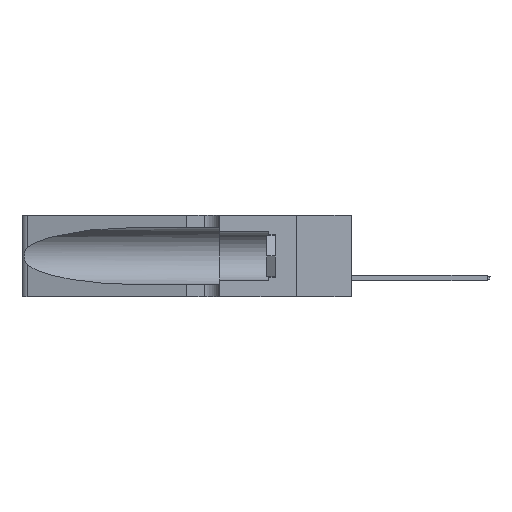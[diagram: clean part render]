
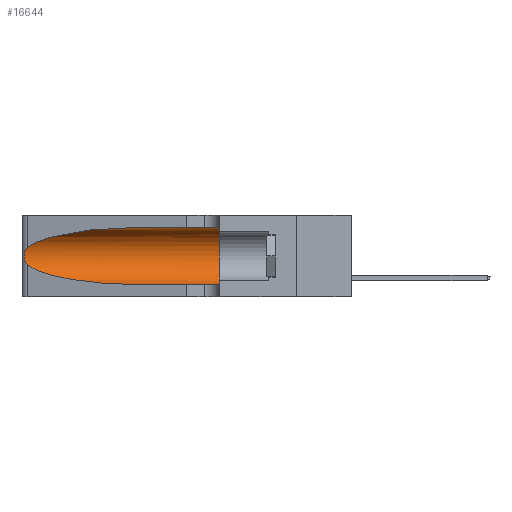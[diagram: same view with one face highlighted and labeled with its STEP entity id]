
A CAD part, left-side view. The second image highlights one B-rep face of the part: STEP entity #16644.
In plain terms, the highlighted cylindrical face has radius 3.308 mm (diameter 6.617 mm), a partial arc.
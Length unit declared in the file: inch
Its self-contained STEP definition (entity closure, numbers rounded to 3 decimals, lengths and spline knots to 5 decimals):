
#372 = CARTESIAN_POINT ( 'NONE',  ( 0.26075, 1.23896, 0.19203 ) ) ;
#516 = CARTESIAN_POINT ( 'NONE',  ( 0.25639, 1.23186, 0.15144 ) ) ;
#840 = ORIENTED_EDGE ( 'NONE', *, *, #10818, .T. ) ;
#975 =( BOUNDED_CURVE ( )  B_SPLINE_CURVE ( 3, ( #2878, #42233, #29083, #22232 ),
 .UNSPECIFIED., .F., .T. ) 
 B_SPLINE_CURVE_WITH_KNOTS ( ( 4, 4 ),
 ( 1.5708, 2.84003 ),
 .UNSPECIFIED. ) 
 CURVE ( )  GEOMETRIC_REPRESENTATION_ITEM ( )  RATIONAL_B_SPLINE_CURVE ( ( 1., 0.87, 0.87, 1. ) ) 
 REPRESENTATION_ITEM ( '' )  );
#1677 = ORIENTED_EDGE ( 'NONE', *, *, #20433, .F. ) ;
#1687 = VERTEX_POINT ( 'NONE', #42105 ) ;
#1975 = EDGE_CURVE ( 'NONE', #4894, #34701, #31952, .T. ) ;
#2878 = CARTESIAN_POINT ( 'NONE',  ( 0.1305, 0.72297, 0.31525 ) ) ;
#3048 = LINE ( 'NONE', #25439, #32761 ) ;
#3253 = CYLINDRICAL_SURFACE ( 'NONE', #29663, 0.13025 ) ;
#4140 = B_SPLINE_CURVE_WITH_KNOTS ( 'NONE', 3,
 ( #6742, #32610, #23046, #16781, #13042, #39171, #372, #6432, #39470, #6877, #10153, #516, #13479, #16913 ),
 .UNSPECIFIED., .F., .F.,
 ( 4, 2, 2, 2, 2, 2, 4 ),
 ( 0., 0.00027, 0.00053, 0.00107, 0.0016, 0.00187, 0.00214 ),
 .UNSPECIFIED. ) ;
#4601 = CARTESIAN_POINT ( 'NONE',  ( 0.25487, 1.22718, 0.14631 ) ) ;
#4681 = CIRCLE ( 'NONE', #40272, 0.13025 ) ;
#4894 = VERTEX_POINT ( 'NONE', #21392 ) ;
#6432 = CARTESIAN_POINT ( 'NONE',  ( 0.26075, 1.23896, 0.178 ) ) ;
#6742 = CARTESIAN_POINT ( 'NONE',  ( 0.25487, 1.22718, 0.22369 ) ) ;
#6877 = CARTESIAN_POINT ( 'NONE',  ( 0.25856, 1.23593, 0.16098 ) ) ;
#10153 = CARTESIAN_POINT ( 'NONE',  ( 0.25789, 1.23486, 0.15765 ) ) ;
#10818 = EDGE_CURVE ( 'NONE', #14510, #4894, #4140, .T. ) ;
#10840 = ORIENTED_EDGE ( 'NONE', *, *, #11871, .T. ) ;
#10971 = CARTESIAN_POINT ( 'NONE',  ( 0.1305, 1.61858, 0.05475 ) ) ;
#11411 = CARTESIAN_POINT ( 'NONE',  ( 0.1305, 0.35, 0.185 ) ) ;
#11726 = DIRECTION ( 'NONE',  ( 0., 0., -1. ) ) ;
#11863 = CARTESIAN_POINT ( 'NONE',  ( 0.1305, 1.61858, 0.185 ) ) ;
#11871 = EDGE_CURVE ( 'NONE', #34701, #22027, #39004, .T. ) ;
#13042 = CARTESIAN_POINT ( 'NONE',  ( 0.25854, 1.2359, 0.20912 ) ) ;
#13290 = ORIENTED_EDGE ( 'NONE', *, *, #18669, .F. ) ;
#13479 = CARTESIAN_POINT ( 'NONE',  ( 0.25555, 1.22993, 0.14849 ) ) ;
#14510 = VERTEX_POINT ( 'NONE', #24016 ) ;
#16044 = VECTOR ( 'NONE', #37000, 39.37008 ) ;
#16644 = ADVANCED_FACE ( 'NONE', ( #39100 ), #3253, .F. ) ;
#16781 = CARTESIAN_POINT ( 'NONE',  ( 0.25787, 1.23484, 0.2124 ) ) ;
#16913 = CARTESIAN_POINT ( 'NONE',  ( 0.25487, 1.22718, 0.14631 ) ) ;
#18001 = ORIENTED_EDGE ( 'NONE', *, *, #1975, .T. ) ;
#18669 = EDGE_CURVE ( 'NONE', #1687, #34874, #3048, .T. ) ;
#19217 = CARTESIAN_POINT ( 'NONE',  ( 0.1305, 0.35, 0.05475 ) ) ;
#19329 = EDGE_LOOP ( 'NONE', ( #24964, #840, #18001, #10840, #1677, #13290 ) ) ;
#20433 = EDGE_CURVE ( 'NONE', #34874, #22027, #4681, .T. ) ;
#21392 = CARTESIAN_POINT ( 'NONE',  ( 0.25487, 1.22718, 0.14631 ) ) ;
#22027 = VERTEX_POINT ( 'NONE', #19217 ) ;
#22232 = CARTESIAN_POINT ( 'NONE',  ( 0.25487, 1.22718, 0.22369 ) ) ;
#23046 = CARTESIAN_POINT ( 'NONE',  ( 0.25639, 1.23184, 0.21858 ) ) ;
#24016 = CARTESIAN_POINT ( 'NONE',  ( 0.25487, 1.22718, 0.22369 ) ) ;
#24964 = ORIENTED_EDGE ( 'NONE', *, *, #34944, .T. ) ;
#25147 = DIRECTION ( 'NONE',  ( 0., -1., 0. ) ) ;
#25439 = CARTESIAN_POINT ( 'NONE',  ( 0.1305, 1.61858, 0.31525 ) ) ;
#27482 = CARTESIAN_POINT ( 'NONE',  ( 0.1305, 0.72297, 0.05475 ) ) ;
#29083 = CARTESIAN_POINT ( 'NONE',  ( 0.2373, 1.15595, 0.28018 ) ) ;
#29663 = AXIS2_PLACEMENT_3D ( 'NONE', #11863, #25147, #11726 ) ;
#31628 = CARTESIAN_POINT ( 'NONE',  ( 0.2373, 1.15595, 0.08982 ) ) ;
#31952 =( BOUNDED_CURVE ( )  B_SPLINE_CURVE ( 3, ( #4601, #31628, #41517, #27482 ),
 .UNSPECIFIED., .F., .T. ) 
 B_SPLINE_CURVE_WITH_KNOTS ( ( 4, 4 ),
 ( 3.44316, 4.71239 ),
 .UNSPECIFIED. ) 
 CURVE ( )  GEOMETRIC_REPRESENTATION_ITEM ( )  RATIONAL_B_SPLINE_CURVE ( ( 1., 0.87, 0.87, 1. ) ) 
 REPRESENTATION_ITEM ( '' )  );
#32610 = CARTESIAN_POINT ( 'NONE',  ( 0.25555, 1.22994, 0.2215 ) ) ;
#32761 = VECTOR ( 'NONE', #38574, 39.37008 ) ;
#34026 = DIRECTION ( 'NONE',  ( 0., 1., 0. ) ) ;
#34701 = VERTEX_POINT ( 'NONE', #40541 ) ;
#34874 = VERTEX_POINT ( 'NONE', #38919 ) ;
#34944 = EDGE_CURVE ( 'NONE', #1687, #14510, #975, .T. ) ;
#37000 = DIRECTION ( 'NONE',  ( 0., -1., 0. ) ) ;
#38574 = DIRECTION ( 'NONE',  ( 0., -1., 0. ) ) ;
#38919 = CARTESIAN_POINT ( 'NONE',  ( 0.1305, 0.35, 0.31525 ) ) ;
#39004 = LINE ( 'NONE', #10971, #16044 ) ;
#39100 = FACE_OUTER_BOUND ( 'NONE', #19329, .T. ) ;
#39171 = CARTESIAN_POINT ( 'NONE',  ( 0.26018, 1.23835, 0.19895 ) ) ;
#39470 = CARTESIAN_POINT ( 'NONE',  ( 0.26017, 1.23833, 0.17102 ) ) ;
#40272 = AXIS2_PLACEMENT_3D ( 'NONE', #11411, #34026, #40474 ) ;
#40474 = DIRECTION ( 'NONE',  ( 0., 0., 1. ) ) ;
#40541 = CARTESIAN_POINT ( 'NONE',  ( 0.1305, 0.72297, 0.05475 ) ) ;
#41517 = CARTESIAN_POINT ( 'NONE',  ( 0.18966, 0.96281, 0.05475 ) ) ;
#42105 = CARTESIAN_POINT ( 'NONE',  ( 0.1305, 0.72297, 0.31525 ) ) ;
#42233 = CARTESIAN_POINT ( 'NONE',  ( 0.18966, 0.96281, 0.31525 ) ) ;
